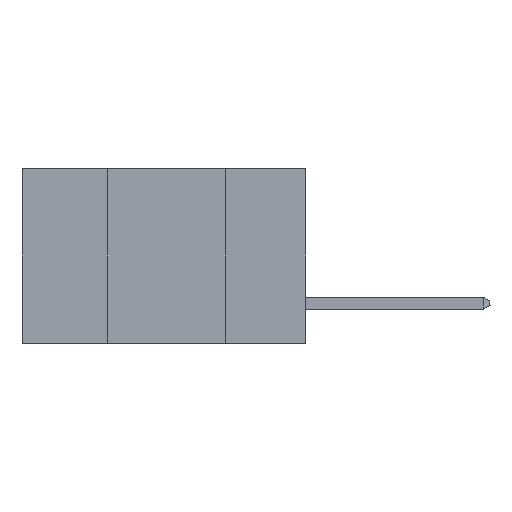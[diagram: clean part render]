
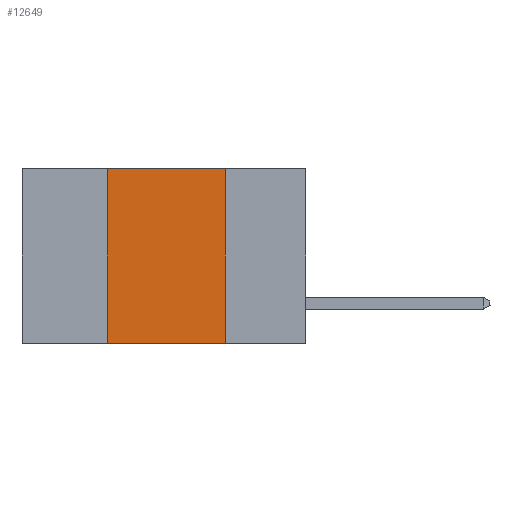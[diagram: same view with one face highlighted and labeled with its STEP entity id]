
A CAD part, left-side view. The second image highlights one B-rep face of the part: STEP entity #12649.
In plain terms, the highlighted planar face has unit normal (-1, 0, 0).
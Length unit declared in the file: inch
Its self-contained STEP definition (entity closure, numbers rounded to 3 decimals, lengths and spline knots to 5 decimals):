
#974 = VECTOR ( 'NONE', #8332, 39.37008 ) ;
#1267 = EDGE_CURVE ( 'NONE', #19170, #1664, #10653, .T. ) ;
#1664 = VERTEX_POINT ( 'NONE', #7514 ) ;
#1779 = VECTOR ( 'NONE', #15187, 39.37008 ) ;
#2656 = DIRECTION ( 'NONE',  ( 0., 0., -1. ) ) ;
#3797 = EDGE_CURVE ( 'NONE', #1664, #11030, #4460, .T. ) ;
#4460 = LINE ( 'NONE', #6994, #974 ) ;
#4833 = EDGE_CURVE ( 'NONE', #19170, #14937, #16178, .T. ) ;
#4977 = ORIENTED_EDGE ( 'NONE', *, *, #4833, .T. ) ;
#5060 = CARTESIAN_POINT ( 'NONE',  ( 0., 0.42, 0. ) ) ;
#6075 = AXIS2_PLACEMENT_3D ( 'NONE', #21623, #7798, #11254 ) ;
#6556 = VECTOR ( 'NONE', #11629, 39.37008 ) ;
#6994 = CARTESIAN_POINT ( 'NONE',  ( 0., 0.6, 0. ) ) ;
#7514 = CARTESIAN_POINT ( 'NONE',  ( 0., 0.42, 0. ) ) ;
#7798 = DIRECTION ( 'NONE',  ( 1., 0., 0. ) ) ;
#7875 = PLANE ( 'NONE',  #6075 ) ;
#8332 = DIRECTION ( 'NONE',  ( 0., -1., 0. ) ) ;
#9482 = EDGE_LOOP ( 'NONE', ( #21944, #10813, #9630, #4977 ) ) ;
#9630 = ORIENTED_EDGE ( 'NONE', *, *, #1267, .F. ) ;
#10653 = LINE ( 'NONE', #5060, #1779 ) ;
#10718 = EDGE_CURVE ( 'NONE', #11030, #14937, #16118, .T. ) ;
#10813 = ORIENTED_EDGE ( 'NONE', *, *, #3797, .F. ) ;
#11030 = VERTEX_POINT ( 'NONE', #11545 ) ;
#11254 = DIRECTION ( 'NONE',  ( 0., 0., -1. ) ) ;
#11493 = CARTESIAN_POINT ( 'NONE',  ( 0., 0.6, -0.37 ) ) ;
#11545 = CARTESIAN_POINT ( 'NONE',  ( 0., 0.17, 0. ) ) ;
#11629 = DIRECTION ( 'NONE',  ( 0., -1., 0. ) ) ;
#12649 = ADVANCED_FACE ( 'NONE', ( #16841 ), #7875, .F. ) ;
#14937 = VERTEX_POINT ( 'NONE', #21075 ) ;
#15187 = DIRECTION ( 'NONE',  ( 0., 0., 1. ) ) ;
#16118 = LINE ( 'NONE', #16421, #21164 ) ;
#16178 = LINE ( 'NONE', #11493, #6556 ) ;
#16421 = CARTESIAN_POINT ( 'NONE',  ( 0., 0.17, 0. ) ) ;
#16454 = CARTESIAN_POINT ( 'NONE',  ( 0., 0.42, -0.37 ) ) ;
#16841 = FACE_OUTER_BOUND ( 'NONE', #9482, .T. ) ;
#19170 = VERTEX_POINT ( 'NONE', #16454 ) ;
#21075 = CARTESIAN_POINT ( 'NONE',  ( 0., 0.17, -0.37 ) ) ;
#21164 = VECTOR ( 'NONE', #2656, 39.37008 ) ;
#21623 = CARTESIAN_POINT ( 'NONE',  ( 0., 0.6, 0. ) ) ;
#21944 = ORIENTED_EDGE ( 'NONE', *, *, #10718, .F. ) ;
